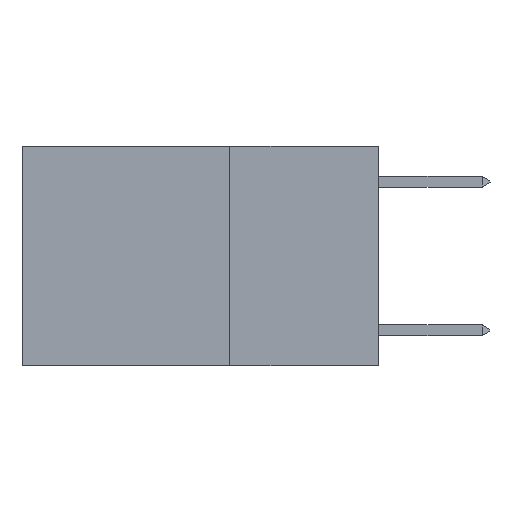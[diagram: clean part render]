
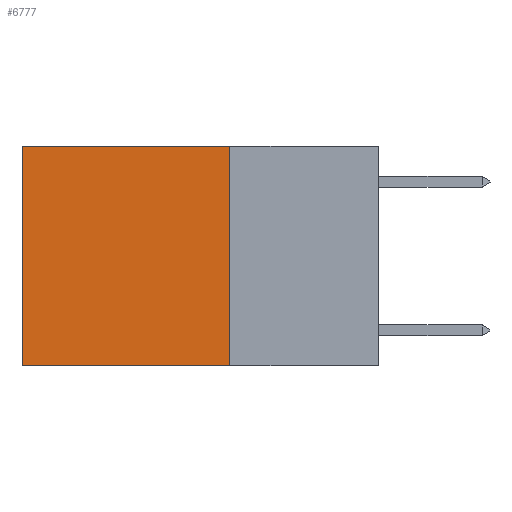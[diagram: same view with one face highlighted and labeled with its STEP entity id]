
A CAD part, left-side view. The second image highlights one B-rep face of the part: STEP entity #6777.
In plain terms, the highlighted planar face has unit normal (-1, 0, 0).
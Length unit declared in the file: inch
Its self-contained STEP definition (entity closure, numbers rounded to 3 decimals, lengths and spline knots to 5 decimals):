
#16 = LINE ( 'NONE', #15738, #11888 ) ;
#86 = DIRECTION ( 'NONE',  ( 0., 0., -1. ) ) ;
#993 = ORIENTED_EDGE ( 'NONE', *, *, #8082, .T. ) ;
#1378 = FACE_OUTER_BOUND ( 'NONE', #19647, .T. ) ;
#2066 = CARTESIAN_POINT ( 'NONE',  ( 0.2625, 0.25, -0.37 ) ) ;
#3460 = LINE ( 'NONE', #19409, #9711 ) ;
#4052 = VERTEX_POINT ( 'NONE', #2066 ) ;
#4352 = VERTEX_POINT ( 'NONE', #9788 ) ;
#4743 = ORIENTED_EDGE ( 'NONE', *, *, #10653, .T. ) ;
#4836 = DIRECTION ( 'NONE',  ( 0., 1., 0. ) ) ;
#6039 = CARTESIAN_POINT ( 'NONE',  ( 0.2625, 0.6, 0. ) ) ;
#6055 = VERTEX_POINT ( 'NONE', #6039 ) ;
#6777 = ADVANCED_FACE ( 'NONE', ( #1378 ), #14199, .F. ) ;
#7198 = VECTOR ( 'NONE', #86, 39.37008 ) ;
#7998 = DIRECTION ( 'NONE',  ( 1., 0., 0. ) ) ;
#8082 = EDGE_CURVE ( 'NONE', #4352, #6055, #13886, .T. ) ;
#9711 = VECTOR ( 'NONE', #12710, 39.37008 ) ;
#9788 = CARTESIAN_POINT ( 'NONE',  ( 0.2625, 0.25, 0. ) ) ;
#10125 = LINE ( 'NONE', #14673, #7198 ) ;
#10653 = EDGE_CURVE ( 'NONE', #6055, #15265, #10125, .T. ) ;
#10721 = CARTESIAN_POINT ( 'NONE',  ( 0.2625, 0.25, 0. ) ) ;
#11720 = EDGE_CURVE ( 'NONE', #4052, #15265, #16, .T. ) ;
#11888 = VECTOR ( 'NONE', #4836, 39.37008 ) ;
#12710 = DIRECTION ( 'NONE',  ( 0., 0., -1. ) ) ;
#13567 = DIRECTION ( 'NONE',  ( 0., 1., 0. ) ) ;
#13886 = LINE ( 'NONE', #10721, #18890 ) ;
#14199 = PLANE ( 'NONE',  #16491 ) ;
#14673 = CARTESIAN_POINT ( 'NONE',  ( 0.2625, 0.6, 0. ) ) ;
#14828 = EDGE_CURVE ( 'NONE', #4352, #4052, #3460, .T. ) ;
#15265 = VERTEX_POINT ( 'NONE', #15722 ) ;
#15537 = ORIENTED_EDGE ( 'NONE', *, *, #11720, .F. ) ;
#15722 = CARTESIAN_POINT ( 'NONE',  ( 0.2625, 0.6, -0.37 ) ) ;
#15738 = CARTESIAN_POINT ( 'NONE',  ( 0.2625, 0.25, -0.37 ) ) ;
#15959 = CARTESIAN_POINT ( 'NONE',  ( 0.2625, 0.25, 0. ) ) ;
#16491 = AXIS2_PLACEMENT_3D ( 'NONE', #15959, #7998, #18989 ) ;
#18449 = ORIENTED_EDGE ( 'NONE', *, *, #14828, .F. ) ;
#18890 = VECTOR ( 'NONE', #13567, 39.37008 ) ;
#18989 = DIRECTION ( 'NONE',  ( 0., 0., -1. ) ) ;
#19409 = CARTESIAN_POINT ( 'NONE',  ( 0.2625, 0.25, 0. ) ) ;
#19647 = EDGE_LOOP ( 'NONE', ( #4743, #15537, #18449, #993 ) ) ;
